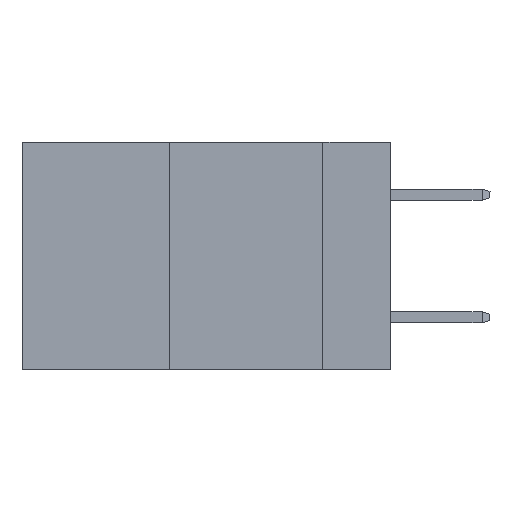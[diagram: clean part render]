
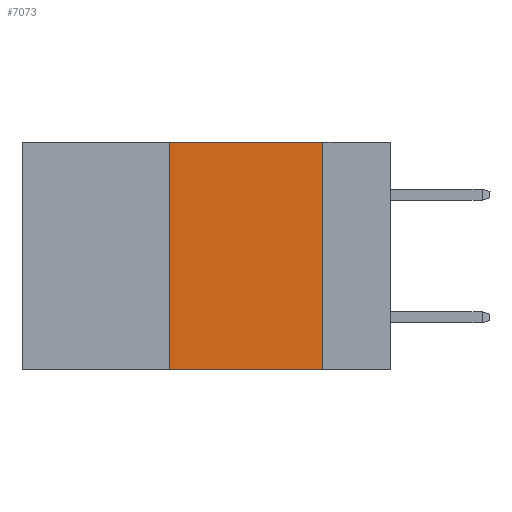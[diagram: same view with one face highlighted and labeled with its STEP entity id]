
A CAD part, left-side view. The second image highlights one B-rep face of the part: STEP entity #7073.
In plain terms, the highlighted planar face has unit normal (-1, 0, 0).
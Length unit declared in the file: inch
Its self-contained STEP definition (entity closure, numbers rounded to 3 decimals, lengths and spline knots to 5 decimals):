
#279 = DIRECTION ( 'NONE',  ( 0., 0., -1. ) ) ;
#290 = ORIENTED_EDGE ( 'NONE', *, *, #4140, .F. ) ;
#513 = CARTESIAN_POINT ( 'NONE',  ( 0., 0.6, -0.37 ) ) ;
#1529 = VECTOR ( 'NONE', #9170, 39.37008 ) ;
#1549 = CARTESIAN_POINT ( 'NONE',  ( 0., 0.11, 0. ) ) ;
#2084 = LINE ( 'NONE', #5524, #5035 ) ;
#2188 = EDGE_CURVE ( 'NONE', #9098, #10458, #2084, .T. ) ;
#2652 = CARTESIAN_POINT ( 'NONE',  ( 0., 0.11, 0. ) ) ;
#3133 = DIRECTION ( 'NONE',  ( 0., 0., 1. ) ) ;
#3441 = EDGE_CURVE ( 'NONE', #15430, #5923, #14264, .T. ) ;
#3574 = LINE ( 'NONE', #1549, #6483 ) ;
#4015 = ORIENTED_EDGE ( 'NONE', *, *, #3441, .T. ) ;
#4140 = EDGE_CURVE ( 'NONE', #15430, #9098, #6600, .T. ) ;
#4786 = EDGE_LOOP ( 'NONE', ( #6834, #7326, #290, #4015 ) ) ;
#5035 = VECTOR ( 'NONE', #7992, 39.37008 ) ;
#5524 = CARTESIAN_POINT ( 'NONE',  ( 0., 0.6, 0. ) ) ;
#5923 = VERTEX_POINT ( 'NONE', #12246 ) ;
#6483 = VECTOR ( 'NONE', #279, 39.37008 ) ;
#6518 = FACE_OUTER_BOUND ( 'NONE', #4786, .T. ) ;
#6600 = LINE ( 'NONE', #14923, #11730 ) ;
#6834 = ORIENTED_EDGE ( 'NONE', *, *, #7949, .F. ) ;
#7073 = ADVANCED_FACE ( 'NONE', ( #6518 ), #7192, .F. ) ;
#7192 = PLANE ( 'NONE',  #15150 ) ;
#7326 = ORIENTED_EDGE ( 'NONE', *, *, #2188, .F. ) ;
#7949 = EDGE_CURVE ( 'NONE', #10458, #5923, #3574, .T. ) ;
#7992 = DIRECTION ( 'NONE',  ( 0., -1., 0. ) ) ;
#8391 = DIRECTION ( 'NONE',  ( 0., 0., -1. ) ) ;
#9098 = VERTEX_POINT ( 'NONE', #13154 ) ;
#9170 = DIRECTION ( 'NONE',  ( 0., -1., 0. ) ) ;
#10458 = VERTEX_POINT ( 'NONE', #2652 ) ;
#10676 = CARTESIAN_POINT ( 'NONE',  ( 0., 0.6, 0. ) ) ;
#11730 = VECTOR ( 'NONE', #3133, 39.37008 ) ;
#11850 = CARTESIAN_POINT ( 'NONE',  ( 0., 0.36, -0.37 ) ) ;
#12246 = CARTESIAN_POINT ( 'NONE',  ( 0., 0.11, -0.37 ) ) ;
#13154 = CARTESIAN_POINT ( 'NONE',  ( 0., 0.36, 0. ) ) ;
#14264 = LINE ( 'NONE', #513, #1529 ) ;
#14923 = CARTESIAN_POINT ( 'NONE',  ( 0., 0.36, 0. ) ) ;
#15150 = AXIS2_PLACEMENT_3D ( 'NONE', #10676, #15261, #8391 ) ;
#15261 = DIRECTION ( 'NONE',  ( 1., 0., 0. ) ) ;
#15430 = VERTEX_POINT ( 'NONE', #11850 ) ;
